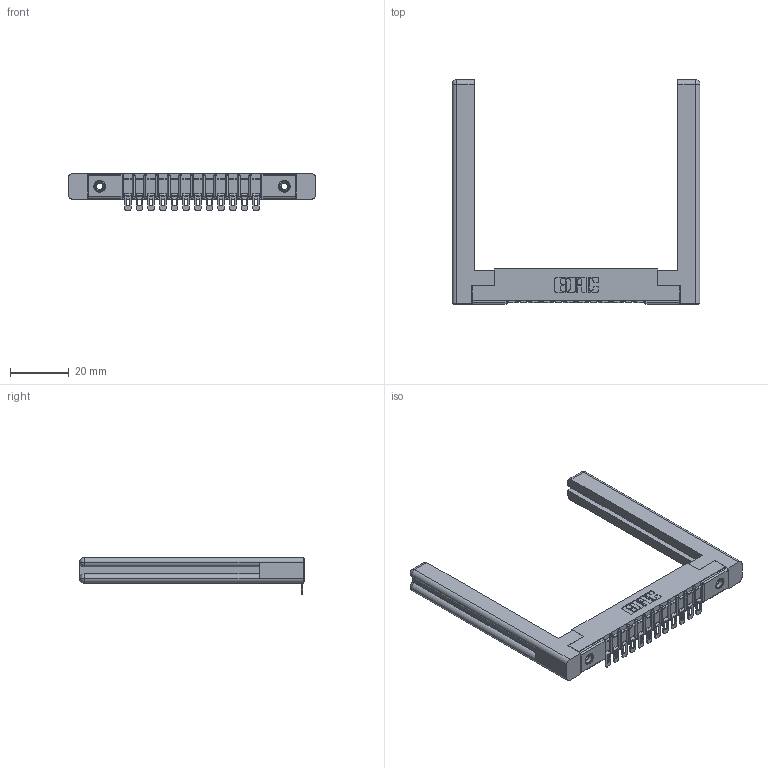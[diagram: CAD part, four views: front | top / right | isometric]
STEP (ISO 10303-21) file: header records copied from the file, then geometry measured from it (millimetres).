
FILE_DESCRIPTION (( 'STEP AP203' ), '1' );
FILE_NAME ('357-012-454-158.STEP', '2020-09-30T13:07:08', ( '' ), ( '' ), 'SwSTEP 2.0', 'SolidWorks 2020', '' );
FILE_SCHEMA (( 'CONFIG_CONTROL_DESIGN' ));
Length unit declared in the file: inch
Products named in the file (5): 345-250-001_345-250-001-102; 307-290-002_554; 357-012-454-158; 307-220-058; 307 Part_.156 Dia Mounting Holes
Assembly tree (17 placements, depth 2):
  357-012-454-158
    307 Part_.156 Dia Mounting Holes
    307-290-002_554  x12
    307-220-058  x2
    345-250-001_345-250-001-102  x2
Bounding box: 84.18 x 76.33 x 12.52 mm (x, y, z)
Volume: 13234.5 mm3; surface area: 14623.5 mm2
Topology: 17 solids, 17 shells, 1245 faces, 3713 edges, 2426 vertices
Faces by surface type: plane 706, cylinder 489, sphere 26, torus 12, cone 12
Entity records: 17584 total; most frequent: CARTESIAN_POINT 2969, ORIENTED_EDGE 2898, DIRECTION 2865, EDGE_CURVE 1449, LINE 1085, VECTOR 1085, VERTEX_POINT 940, AXIS2_PLACEMENT_3D 890
